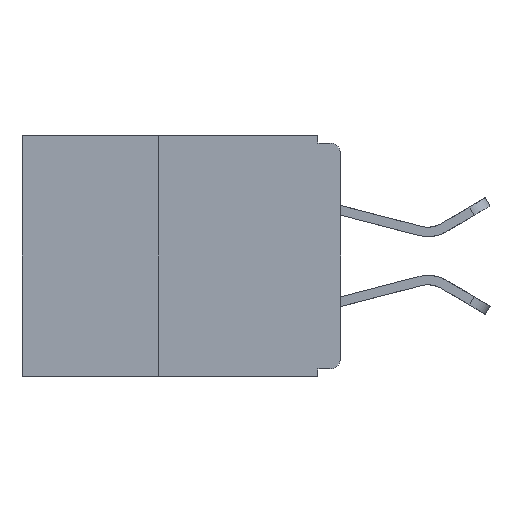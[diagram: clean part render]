
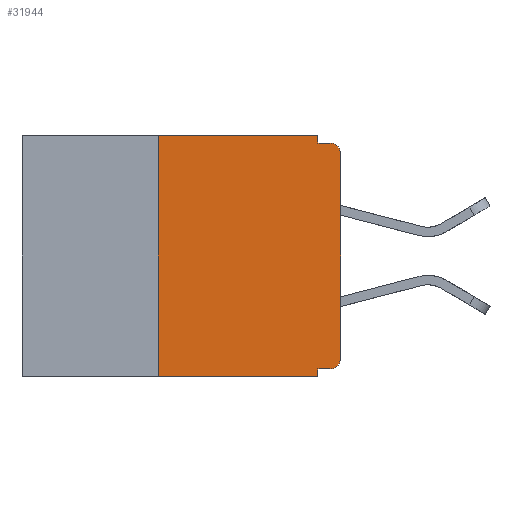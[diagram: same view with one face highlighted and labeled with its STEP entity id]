
A CAD part, left-side view. The second image highlights one B-rep face of the part: STEP entity #31944.
In plain terms, the highlighted planar face has unit normal (-1, 0, 0).
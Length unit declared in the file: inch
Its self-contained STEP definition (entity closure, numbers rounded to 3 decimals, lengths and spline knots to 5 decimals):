
#595 = VERTEX_POINT ( 'NONE', #20665 ) ;
#706 = CARTESIAN_POINT ( 'NONE',  ( 0., 0., -0.32 ) ) ;
#754 = CIRCLE ( 'NONE', #31492, 0.015 ) ;
#1312 = DIRECTION ( 'NONE',  ( 0., 0., -1. ) ) ;
#1897 = LINE ( 'NONE', #20529, #20822 ) ;
#3127 = DIRECTION ( 'NONE',  ( 0., -1., 0. ) ) ;
#3701 = LINE ( 'NONE', #4827, #9097 ) ;
#4182 = CARTESIAN_POINT ( 'NONE',  ( 0., 0.031, -0.33 ) ) ;
#4469 = CARTESIAN_POINT ( 'NONE',  ( 0., 0., -0.025 ) ) ;
#4576 = DIRECTION ( 'NONE',  ( -1., 0., 0. ) ) ;
#4827 = CARTESIAN_POINT ( 'NONE',  ( 0., 0.437, 0. ) ) ;
#5699 = CARTESIAN_POINT ( 'NONE',  ( 0., 0., -0.01 ) ) ;
#5854 = LINE ( 'NONE', #706, #26968 ) ;
#6239 = DIRECTION ( 'NONE',  ( -1., 0., 0. ) ) ;
#6327 = CARTESIAN_POINT ( 'NONE',  ( 0., 0.25, -0.33 ) ) ;
#7411 = DIRECTION ( 'NONE',  ( 0., -1., 0. ) ) ;
#7986 = LINE ( 'NONE', #5699, #20719 ) ;
#8024 = VERTEX_POINT ( 'NONE', #23667 ) ;
#8186 = ORIENTED_EDGE ( 'NONE', *, *, #19488, .T. ) ;
#9097 = VECTOR ( 'NONE', #7411, 39.37008 ) ;
#10129 = CARTESIAN_POINT ( 'NONE',  ( 0., 0.25, 0. ) ) ;
#10378 = VERTEX_POINT ( 'NONE', #10742 ) ;
#10520 = VECTOR ( 'NONE', #14480, 39.37008 ) ;
#10526 = ORIENTED_EDGE ( 'NONE', *, *, #32396, .F. ) ;
#10539 = LINE ( 'NONE', #6327, #23972 ) ;
#10742 = CARTESIAN_POINT ( 'NONE',  ( 0., 0.031, -0.33 ) ) ;
#11131 = CIRCLE ( 'NONE', #13319, 0.015 ) ;
#13319 = AXIS2_PLACEMENT_3D ( 'NONE', #20014, #4576, #22556 ) ;
#14330 = CARTESIAN_POINT ( 'NONE',  ( 0., 0.437, 0. ) ) ;
#14480 = DIRECTION ( 'NONE',  ( 0., 0., -1. ) ) ;
#15343 = DIRECTION ( 'NONE',  ( 0., 0., 1. ) ) ;
#15485 = CARTESIAN_POINT ( 'NONE',  ( 0., 0.031, -0.32 ) ) ;
#16157 = EDGE_CURVE ( 'NONE', #25050, #26743, #3701, .T. ) ;
#16913 = DIRECTION ( 'NONE',  ( 1., 0., 0. ) ) ;
#17784 = EDGE_LOOP ( 'NONE', ( #20870, #25506, #24341, #31756, #32196, #19798, #8186, #30434, #10526, #30973 ) ) ;
#18176 = CARTESIAN_POINT ( 'NONE',  ( 0., 0.031, -0.01 ) ) ;
#18511 = VERTEX_POINT ( 'NONE', #32621 ) ;
#18715 = VECTOR ( 'NONE', #15343, 39.37008 ) ;
#18809 = DIRECTION ( 'NONE',  ( 0., 1., 0. ) ) ;
#19488 = EDGE_CURVE ( 'NONE', #20000, #10378, #1897, .T. ) ;
#19631 = DIRECTION ( 'NONE',  ( 0., 0., -1. ) ) ;
#19795 = CARTESIAN_POINT ( 'NONE',  ( 0., 0.031, 0. ) ) ;
#19798 = ORIENTED_EDGE ( 'NONE', *, *, #23854, .F. ) ;
#19831 = EDGE_CURVE ( 'NONE', #26743, #32251, #31446, .T. ) ;
#20000 = VERTEX_POINT ( 'NONE', #27664 ) ;
#20014 = CARTESIAN_POINT ( 'NONE',  ( 0., 0.015, -0.305 ) ) ;
#20529 = CARTESIAN_POINT ( 'NONE',  ( 0., 0.437, -0.33 ) ) ;
#20571 = EDGE_CURVE ( 'NONE', #595, #23567, #25393, .T. ) ;
#20665 = CARTESIAN_POINT ( 'NONE',  ( 0., 0., -0.305 ) ) ;
#20719 = VECTOR ( 'NONE', #3127, 39.37008 ) ;
#20822 = VECTOR ( 'NONE', #30660, 39.37008 ) ;
#20870 = ORIENTED_EDGE ( 'NONE', *, *, #20571, .T. ) ;
#21541 = CARTESIAN_POINT ( 'NONE',  ( 0., 0.015, -0.025 ) ) ;
#22422 = VERTEX_POINT ( 'NONE', #15485 ) ;
#22556 = DIRECTION ( 'NONE',  ( 0., 0., -1. ) ) ;
#23567 = VERTEX_POINT ( 'NONE', #4469 ) ;
#23667 = CARTESIAN_POINT ( 'NONE',  ( 0., 0.015, -0.01 ) ) ;
#23854 = EDGE_CURVE ( 'NONE', #20000, #25050, #10539, .T. ) ;
#23972 = VECTOR ( 'NONE', #24159, 39.37008 ) ;
#24072 = DIRECTION ( 'NONE',  ( 0., 0., -1. ) ) ;
#24159 = DIRECTION ( 'NONE',  ( 0., 0., 1. ) ) ;
#24341 = ORIENTED_EDGE ( 'NONE', *, *, #25882, .F. ) ;
#25050 = VERTEX_POINT ( 'NONE', #10129 ) ;
#25393 = LINE ( 'NONE', #30380, #18715 ) ;
#25506 = ORIENTED_EDGE ( 'NONE', *, *, #28859, .T. ) ;
#25882 = EDGE_CURVE ( 'NONE', #32251, #8024, #7986, .T. ) ;
#26225 = LINE ( 'NONE', #4182, #32915 ) ;
#26711 = AXIS2_PLACEMENT_3D ( 'NONE', #14330, #16913, #1312 ) ;
#26743 = VERTEX_POINT ( 'NONE', #19795 ) ;
#26796 = EDGE_CURVE ( 'NONE', #18511, #595, #11131, .T. ) ;
#26857 = PLANE ( 'NONE',  #26711 ) ;
#26968 = VECTOR ( 'NONE', #18809, 39.37008 ) ;
#27664 = CARTESIAN_POINT ( 'NONE',  ( 0., 0.25, -0.33 ) ) ;
#28615 = FACE_OUTER_BOUND ( 'NONE', #17784, .T. ) ;
#28859 = EDGE_CURVE ( 'NONE', #23567, #8024, #754, .T. ) ;
#30380 = CARTESIAN_POINT ( 'NONE',  ( 0., 0., 0. ) ) ;
#30434 = ORIENTED_EDGE ( 'NONE', *, *, #31513, .F. ) ;
#30660 = DIRECTION ( 'NONE',  ( 0., -1., 0. ) ) ;
#30973 = ORIENTED_EDGE ( 'NONE', *, *, #26796, .T. ) ;
#31446 = LINE ( 'NONE', #32056, #10520 ) ;
#31492 = AXIS2_PLACEMENT_3D ( 'NONE', #21541, #6239, #24072 ) ;
#31513 = EDGE_CURVE ( 'NONE', #22422, #10378, #26225, .T. ) ;
#31756 = ORIENTED_EDGE ( 'NONE', *, *, #19831, .F. ) ;
#31944 = ADVANCED_FACE ( 'NONE', ( #28615 ), #26857, .F. ) ;
#32056 = CARTESIAN_POINT ( 'NONE',  ( 0., 0.031, 0. ) ) ;
#32196 = ORIENTED_EDGE ( 'NONE', *, *, #16157, .F. ) ;
#32251 = VERTEX_POINT ( 'NONE', #18176 ) ;
#32396 = EDGE_CURVE ( 'NONE', #18511, #22422, #5854, .T. ) ;
#32621 = CARTESIAN_POINT ( 'NONE',  ( 0., 0.015, -0.32 ) ) ;
#32915 = VECTOR ( 'NONE', #19631, 39.37008 ) ;
